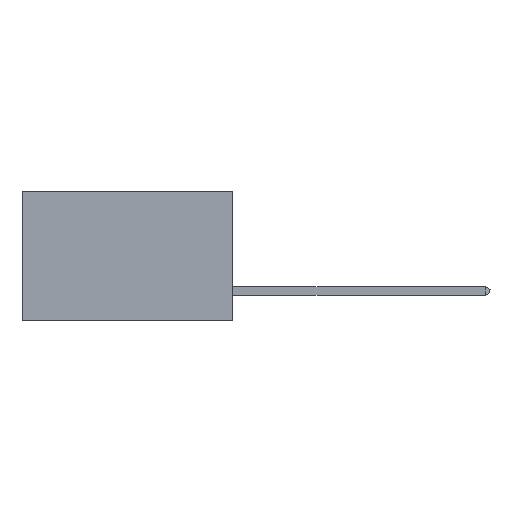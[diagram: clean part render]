
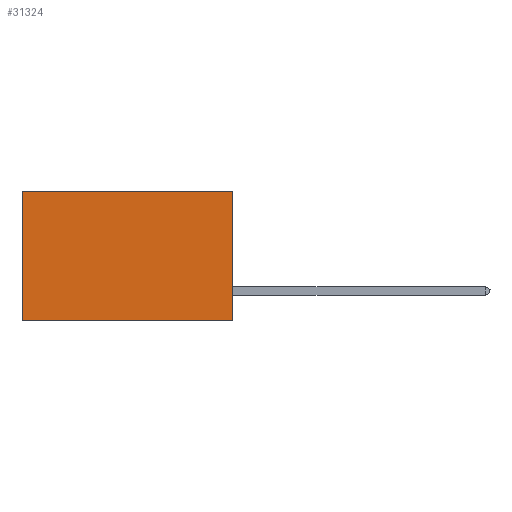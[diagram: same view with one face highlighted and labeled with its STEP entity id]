
A CAD part, left-side view. The second image highlights one B-rep face of the part: STEP entity #31324.
In plain terms, the highlighted planar face has unit normal (-1, 0, 0).
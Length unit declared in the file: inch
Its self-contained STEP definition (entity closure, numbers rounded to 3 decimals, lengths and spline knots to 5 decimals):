
#3798 = LINE ( 'NONE', #23115, #41256 ) ;
#4223 = EDGE_CURVE ( 'NONE', #6402, #34778, #3798, .T. ) ;
#4914 = CARTESIAN_POINT ( 'NONE',  ( 0.2875, 0.6, 0. ) ) ;
#6094 = CARTESIAN_POINT ( 'NONE',  ( 0.2875, 0.6, 0. ) ) ;
#6402 = VERTEX_POINT ( 'NONE', #15453 ) ;
#7525 = DIRECTION ( 'NONE',  ( 1., 0., 0. ) ) ;
#9477 = CARTESIAN_POINT ( 'NONE',  ( 0.2875, 0., -0.37 ) ) ;
#9802 = CARTESIAN_POINT ( 'NONE',  ( 0.2875, 0.6, -0.37 ) ) ;
#10469 = CARTESIAN_POINT ( 'NONE',  ( 0.2875, 0., -0.37 ) ) ;
#11659 = VECTOR ( 'NONE', #36199, 39.37008 ) ;
#12192 = DIRECTION ( 'NONE',  ( 0., 0., -1. ) ) ;
#13344 = EDGE_CURVE ( 'NONE', #6402, #37675, #36103, .T. ) ;
#14421 = ORIENTED_EDGE ( 'NONE', *, *, #4223, .F. ) ;
#15453 = CARTESIAN_POINT ( 'NONE',  ( 0.2875, 0., 0. ) ) ;
#16194 = FACE_OUTER_BOUND ( 'NONE', #36535, .T. ) ;
#16389 = DIRECTION ( 'NONE',  ( 0., 0., -1. ) ) ;
#22159 = EDGE_CURVE ( 'NONE', #34778, #29198, #36394, .T. ) ;
#23115 = CARTESIAN_POINT ( 'NONE',  ( 0.2875, 0., 0. ) ) ;
#27930 = DIRECTION ( 'NONE',  ( 0., 1., 0. ) ) ;
#28175 = PLANE ( 'NONE',  #40663 ) ;
#29198 = VERTEX_POINT ( 'NONE', #9802 ) ;
#29768 = ORIENTED_EDGE ( 'NONE', *, *, #22159, .F. ) ;
#29876 = ORIENTED_EDGE ( 'NONE', *, *, #40330, .T. ) ;
#31090 = CARTESIAN_POINT ( 'NONE',  ( 0.2875, 0., 0. ) ) ;
#31324 = ADVANCED_FACE ( 'NONE', ( #16194 ), #28175, .F. ) ;
#32081 = VECTOR ( 'NONE', #27930, 39.37008 ) ;
#34778 = VERTEX_POINT ( 'NONE', #9477 ) ;
#35188 = CARTESIAN_POINT ( 'NONE',  ( 0.2875, 0., 0. ) ) ;
#36103 = LINE ( 'NONE', #31090, #44158 ) ;
#36199 = DIRECTION ( 'NONE',  ( 0., 0., -1. ) ) ;
#36394 = LINE ( 'NONE', #10469, #32081 ) ;
#36535 = EDGE_LOOP ( 'NONE', ( #29876, #29768, #14421, #43723 ) ) ;
#37675 = VERTEX_POINT ( 'NONE', #6094 ) ;
#38963 = LINE ( 'NONE', #4914, #11659 ) ;
#40330 = EDGE_CURVE ( 'NONE', #37675, #29198, #38963, .T. ) ;
#40663 = AXIS2_PLACEMENT_3D ( 'NONE', #35188, #7525, #12192 ) ;
#41256 = VECTOR ( 'NONE', #16389, 39.37008 ) ;
#42418 = DIRECTION ( 'NONE',  ( 0., 1., 0. ) ) ;
#43723 = ORIENTED_EDGE ( 'NONE', *, *, #13344, .T. ) ;
#44158 = VECTOR ( 'NONE', #42418, 39.37008 ) ;
